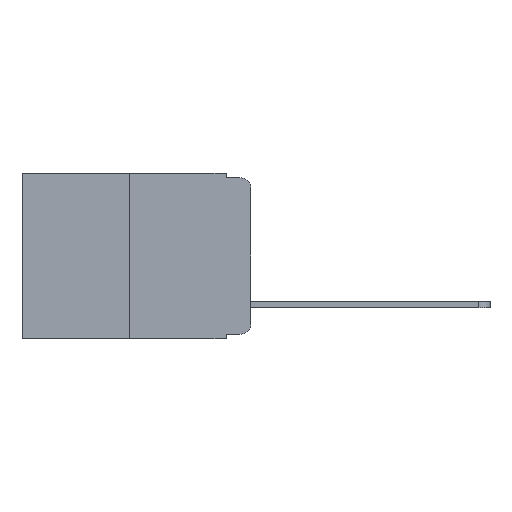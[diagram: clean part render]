
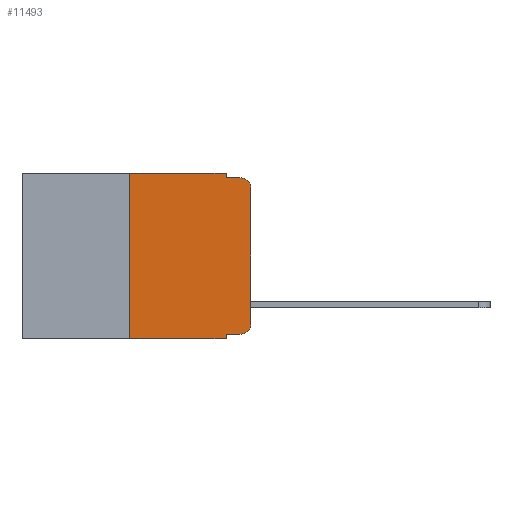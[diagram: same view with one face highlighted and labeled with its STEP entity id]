
A CAD part, left-side view. The second image highlights one B-rep face of the part: STEP entity #11493.
In plain terms, the highlighted planar face has unit normal (-1, 0, 0).
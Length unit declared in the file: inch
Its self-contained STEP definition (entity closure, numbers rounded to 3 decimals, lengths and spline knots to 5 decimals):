
#55 = VERTEX_POINT ( 'NONE', #89 ) ;
#89 = CARTESIAN_POINT ( 'NONE',  ( 0., 0.051, 0. ) ) ;
#118 = CARTESIAN_POINT ( 'NONE',  ( 0., 0.051, 0. ) ) ;
#313 = CARTESIAN_POINT ( 'NONE',  ( 0., 0.051, -0.01 ) ) ;
#401 = VECTOR ( 'NONE', #2279, 39.37008 ) ;
#507 = VERTEX_POINT ( 'NONE', #5073 ) ;
#525 = LINE ( 'NONE', #4837, #4732 ) ;
#725 = ORIENTED_EDGE ( 'NONE', *, *, #3840, .T. ) ;
#883 = ORIENTED_EDGE ( 'NONE', *, *, #10086, .F. ) ;
#1043 = ORIENTED_EDGE ( 'NONE', *, *, #1527, .F. ) ;
#1097 = CARTESIAN_POINT ( 'NONE',  ( 0., 0.473, 0. ) ) ;
#1141 = VERTEX_POINT ( 'NONE', #12661 ) ;
#1286 = CARTESIAN_POINT ( 'NONE',  ( 0., 0., 0. ) ) ;
#1337 = LINE ( 'NONE', #118, #4765 ) ;
#1391 = DIRECTION ( 'NONE',  ( 1., 0., 0. ) ) ;
#1527 = EDGE_CURVE ( 'NONE', #1141, #3740, #1337, .T. ) ;
#1547 = VERTEX_POINT ( 'NONE', #313 ) ;
#1704 = CARTESIAN_POINT ( 'NONE',  ( 0., 0.25, 0. ) ) ;
#1736 = ORIENTED_EDGE ( 'NONE', *, *, #11952, .T. ) ;
#1791 = FACE_OUTER_BOUND ( 'NONE', #9002, .T. ) ;
#2238 = DIRECTION ( 'NONE',  ( 0., 0., -1. ) ) ;
#2251 = VECTOR ( 'NONE', #5614, 39.37008 ) ;
#2279 = DIRECTION ( 'NONE',  ( 0., -1., 0. ) ) ;
#2349 = VECTOR ( 'NONE', #5423, 39.37008 ) ;
#2508 = EDGE_CURVE ( 'NONE', #55, #1547, #525, .T. ) ;
#3063 = VERTEX_POINT ( 'NONE', #3730 ) ;
#3351 = ORIENTED_EDGE ( 'NONE', *, *, #2508, .F. ) ;
#3537 = CARTESIAN_POINT ( 'NONE',  ( 0., 0.473, -0.343 ) ) ;
#3730 = CARTESIAN_POINT ( 'NONE',  ( 0., 0.02, -0.333 ) ) ;
#3740 = VERTEX_POINT ( 'NONE', #10922 ) ;
#3791 = VERTEX_POINT ( 'NONE', #7771 ) ;
#3840 = EDGE_CURVE ( 'NONE', #3791, #11038, #4694, .T. ) ;
#4160 = ORIENTED_EDGE ( 'NONE', *, *, #4405, .F. ) ;
#4405 = EDGE_CURVE ( 'NONE', #11025, #55, #8958, .T. ) ;
#4514 = ORIENTED_EDGE ( 'NONE', *, *, #6523, .T. ) ;
#4528 = PLANE ( 'NONE',  #10510 ) ;
#4635 = VERTEX_POINT ( 'NONE', #10584 ) ;
#4694 = LINE ( 'NONE', #1286, #9975 ) ;
#4732 = VECTOR ( 'NONE', #11113, 39.37008 ) ;
#4765 = VECTOR ( 'NONE', #11095, 39.37008 ) ;
#4837 = CARTESIAN_POINT ( 'NONE',  ( 0., 0.051, 0. ) ) ;
#4861 = ORIENTED_EDGE ( 'NONE', *, *, #7666, .T. ) ;
#5073 = CARTESIAN_POINT ( 'NONE',  ( 0., 0.02, -0.01 ) ) ;
#5305 = DIRECTION ( 'NONE',  ( -1., 0., 0. ) ) ;
#5423 = DIRECTION ( 'NONE',  ( 0., 0., 1. ) ) ;
#5543 = DIRECTION ( 'NONE',  ( 0., 0., -1. ) ) ;
#5614 = DIRECTION ( 'NONE',  ( 0., -1., 0. ) ) ;
#6031 = VECTOR ( 'NONE', #6116, 39.37008 ) ;
#6055 = DIRECTION ( 'NONE',  ( -1., 0., 0. ) ) ;
#6116 = DIRECTION ( 'NONE',  ( 0., -1., 0. ) ) ;
#6150 = CIRCLE ( 'NONE', #12335, 0.02 ) ;
#6263 = VECTOR ( 'NONE', #7566, 39.37008 ) ;
#6353 = CARTESIAN_POINT ( 'NONE',  ( 0., 0.02, -0.313 ) ) ;
#6523 = EDGE_CURVE ( 'NONE', #11038, #507, #8726, .T. ) ;
#6694 = LINE ( 'NONE', #7251, #2349 ) ;
#7251 = CARTESIAN_POINT ( 'NONE',  ( 0., 0.25, 0. ) ) ;
#7298 = CARTESIAN_POINT ( 'NONE',  ( 0., 0.051, -0.333 ) ) ;
#7535 = CARTESIAN_POINT ( 'NONE',  ( 0., 0.051, -0.01 ) ) ;
#7566 = DIRECTION ( 'NONE',  ( 0., -1., 0. ) ) ;
#7666 = EDGE_CURVE ( 'NONE', #1141, #3063, #8944, .T. ) ;
#7771 = CARTESIAN_POINT ( 'NONE',  ( 0., 0., -0.313 ) ) ;
#7906 = EDGE_CURVE ( 'NONE', #1547, #507, #8175, .T. ) ;
#8158 = DIRECTION ( 'NONE',  ( 0., 0., 1. ) ) ;
#8175 = LINE ( 'NONE', #7535, #2251 ) ;
#8315 = ORIENTED_EDGE ( 'NONE', *, *, #12770, .T. ) ;
#8580 = LINE ( 'NONE', #3537, #6263 ) ;
#8684 = AXIS2_PLACEMENT_3D ( 'NONE', #10921, #6055, #10964 ) ;
#8726 = CIRCLE ( 'NONE', #8684, 0.02 ) ;
#8774 = ORIENTED_EDGE ( 'NONE', *, *, #7906, .F. ) ;
#8944 = LINE ( 'NONE', #7298, #401 ) ;
#8958 = LINE ( 'NONE', #1097, #6031 ) ;
#9002 = EDGE_LOOP ( 'NONE', ( #725, #4514, #8774, #3351, #4160, #883, #8315, #1043, #4861, #1736 ) ) ;
#9975 = VECTOR ( 'NONE', #8158, 39.37008 ) ;
#10086 = EDGE_CURVE ( 'NONE', #4635, #11025, #6694, .T. ) ;
#10510 = AXIS2_PLACEMENT_3D ( 'NONE', #11470, #1391, #5543 ) ;
#10511 = CARTESIAN_POINT ( 'NONE',  ( 0., 0., -0.03 ) ) ;
#10584 = CARTESIAN_POINT ( 'NONE',  ( 0., 0.25, -0.343 ) ) ;
#10921 = CARTESIAN_POINT ( 'NONE',  ( 0., 0.02, -0.03 ) ) ;
#10922 = CARTESIAN_POINT ( 'NONE',  ( 0., 0.051, -0.343 ) ) ;
#10964 = DIRECTION ( 'NONE',  ( 0., 0., -1. ) ) ;
#11025 = VERTEX_POINT ( 'NONE', #1704 ) ;
#11038 = VERTEX_POINT ( 'NONE', #10511 ) ;
#11095 = DIRECTION ( 'NONE',  ( 0., 0., -1. ) ) ;
#11113 = DIRECTION ( 'NONE',  ( 0., 0., -1. ) ) ;
#11470 = CARTESIAN_POINT ( 'NONE',  ( 0., 0.473, 0. ) ) ;
#11493 = ADVANCED_FACE ( 'NONE', ( #1791 ), #4528, .F. ) ;
#11952 = EDGE_CURVE ( 'NONE', #3063, #3791, #6150, .T. ) ;
#12335 = AXIS2_PLACEMENT_3D ( 'NONE', #6353, #5305, #2238 ) ;
#12661 = CARTESIAN_POINT ( 'NONE',  ( 0., 0.051, -0.333 ) ) ;
#12770 = EDGE_CURVE ( 'NONE', #4635, #3740, #8580, .T. ) ;
